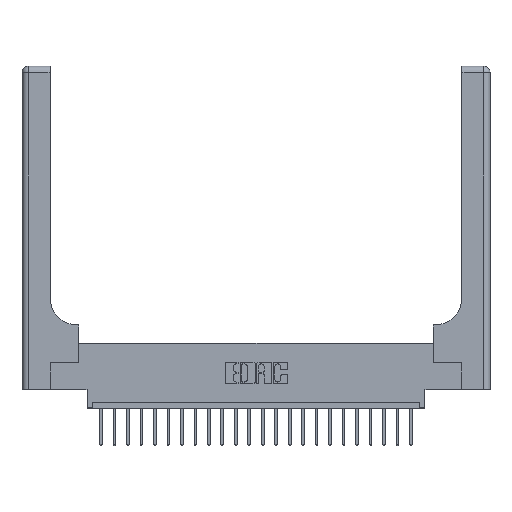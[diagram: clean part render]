
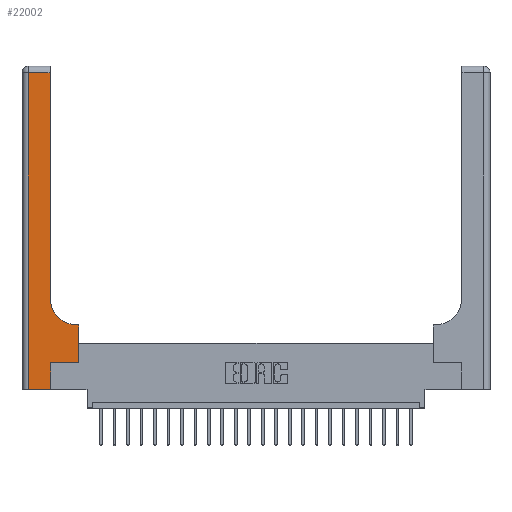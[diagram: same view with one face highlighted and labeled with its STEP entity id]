
A CAD part, top view. The second image highlights one B-rep face of the part: STEP entity #22002.
In plain terms, the highlighted planar face has unit normal (0, 0, 1).
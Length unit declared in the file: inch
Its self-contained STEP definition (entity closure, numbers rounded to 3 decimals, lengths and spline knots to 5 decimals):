
#860 = ORIENTED_EDGE ( 'NONE', *, *, #4540, .T. ) ;
#956 = ORIENTED_EDGE ( 'NONE', *, *, #17757, .T. ) ;
#1184 = EDGE_CURVE ( 'NONE', #16514, #21047, #18964, .T. ) ;
#1452 = CARTESIAN_POINT ( 'NONE',  ( 0.26, 3., 0.37 ) ) ;
#1758 = CARTESIAN_POINT ( 'NONE',  ( 0.528, 0.25, 0.37 ) ) ;
#2264 = DIRECTION ( 'NONE',  ( -1., 0., 0. ) ) ;
#2512 = CARTESIAN_POINT ( 'NONE',  ( 0.51, 0.85, 0.37 ) ) ;
#3030 = VERTEX_POINT ( 'NONE', #13563 ) ;
#3542 = DIRECTION ( 'NONE',  ( 0., 1., 0. ) ) ;
#3850 = EDGE_CURVE ( 'NONE', #17788, #13580, #21428, .T. ) ;
#3981 = CIRCLE ( 'NONE', #13680, 0.25 ) ;
#4122 = LINE ( 'NONE', #12991, #8092 ) ;
#4367 = DIRECTION ( 'NONE',  ( 1., 0., 0. ) ) ;
#4520 = ORIENTED_EDGE ( 'NONE', *, *, #20509, .T. ) ;
#4539 = EDGE_LOOP ( 'NONE', ( #12520, #20703, #9041, #860, #22827, #956, #18592, #10675, #4520 ) ) ;
#4540 = EDGE_CURVE ( 'NONE', #21047, #13183, #22746, .T. ) ;
#4977 = CARTESIAN_POINT ( 'NONE',  ( 0.528, 0.25, 0.37 ) ) ;
#5408 = DIRECTION ( 'NONE',  ( -1., 0., 0. ) ) ;
#5410 = CARTESIAN_POINT ( 'NONE',  ( 0.26, 0.6, 0.37 ) ) ;
#6060 = VECTOR ( 'NONE', #19617, 39.37008 ) ;
#6388 = DIRECTION ( 'NONE',  ( 1., 0., 0. ) ) ;
#7308 = VECTOR ( 'NONE', #6388, 39.37008 ) ;
#7372 = DIRECTION ( 'NONE',  ( 0., 1., 0. ) ) ;
#8092 = VECTOR ( 'NONE', #17781, 39.37008 ) ;
#8501 = AXIS2_PLACEMENT_3D ( 'NONE', #10665, #19775, #5408 ) ;
#8605 = CARTESIAN_POINT ( 'NONE',  ( 0., 0., 0.37 ) ) ;
#8743 = CARTESIAN_POINT ( 'NONE',  ( 0.528, 0.6, 0.37 ) ) ;
#9041 = ORIENTED_EDGE ( 'NONE', *, *, #1184, .T. ) ;
#10665 = CARTESIAN_POINT ( 'NONE',  ( 0., 3., 0.37 ) ) ;
#10675 = ORIENTED_EDGE ( 'NONE', *, *, #3850, .T. ) ;
#12109 = EDGE_CURVE ( 'NONE', #20172, #17788, #12489, .T. ) ;
#12306 = PLANE ( 'NONE',  #8501 ) ;
#12427 = VECTOR ( 'NONE', #7372, 39.37008 ) ;
#12489 = LINE ( 'NONE', #1758, #6060 ) ;
#12520 = ORIENTED_EDGE ( 'NONE', *, *, #20698, .T. ) ;
#12707 = CARTESIAN_POINT ( 'NONE',  ( 0.06, 2.94, 0.37 ) ) ;
#12991 = CARTESIAN_POINT ( 'NONE',  ( 0., 2.94, 0.37 ) ) ;
#13183 = VERTEX_POINT ( 'NONE', #19075 ) ;
#13563 = CARTESIAN_POINT ( 'NONE',  ( 0.26, 0.85, 0.37 ) ) ;
#13580 = VERTEX_POINT ( 'NONE', #21351 ) ;
#13680 = AXIS2_PLACEMENT_3D ( 'NONE', #2512, #20384, #4367 ) ;
#14725 = EDGE_CURVE ( 'NONE', #13183, #22139, #16025, .T. ) ;
#15343 = CARTESIAN_POINT ( 'NONE',  ( 0.06, 3., 0.37 ) ) ;
#15636 = LINE ( 'NONE', #22770, #21496 ) ;
#15750 = DIRECTION ( 'NONE',  ( 1., 0., 0. ) ) ;
#16025 = LINE ( 'NONE', #16253, #12427 ) ;
#16037 = FACE_OUTER_BOUND ( 'NONE', #4539, .T. ) ;
#16253 = CARTESIAN_POINT ( 'NONE',  ( 0.265, 0., 0.37 ) ) ;
#16514 = VERTEX_POINT ( 'NONE', #12707 ) ;
#16557 = CARTESIAN_POINT ( 'NONE',  ( 0.26, 2.94, 0.37 ) ) ;
#17088 = DIRECTION ( 'NONE',  ( 0., -1., 0. ) ) ;
#17695 = VECTOR ( 'NONE', #17088, 39.37008 ) ;
#17757 = EDGE_CURVE ( 'NONE', #22139, #20172, #15636, .T. ) ;
#17781 = DIRECTION ( 'NONE',  ( -1., 0., 0. ) ) ;
#17788 = VERTEX_POINT ( 'NONE', #8743 ) ;
#18592 = ORIENTED_EDGE ( 'NONE', *, *, #12109, .T. ) ;
#18782 = EDGE_CURVE ( 'NONE', #22976, #16514, #4122, .T. ) ;
#18902 = VECTOR ( 'NONE', #2264, 39.37008 ) ;
#18964 = LINE ( 'NONE', #15343, #17695 ) ;
#19075 = CARTESIAN_POINT ( 'NONE',  ( 0.265, 0., 0.37 ) ) ;
#19617 = DIRECTION ( 'NONE',  ( 0., 1., 0. ) ) ;
#19775 = DIRECTION ( 'NONE',  ( 0., 0., -1. ) ) ;
#20172 = VERTEX_POINT ( 'NONE', #4977 ) ;
#20384 = DIRECTION ( 'NONE',  ( 0., 0., -1. ) ) ;
#20509 = EDGE_CURVE ( 'NONE', #13580, #3030, #3981, .T. ) ;
#20698 = EDGE_CURVE ( 'NONE', #3030, #22976, #21070, .T. ) ;
#20703 = ORIENTED_EDGE ( 'NONE', *, *, #18782, .T. ) ;
#21047 = VERTEX_POINT ( 'NONE', #22105 ) ;
#21070 = LINE ( 'NONE', #1452, #22270 ) ;
#21351 = CARTESIAN_POINT ( 'NONE',  ( 0.51, 0.6, 0.37 ) ) ;
#21428 = LINE ( 'NONE', #5410, #18902 ) ;
#21496 = VECTOR ( 'NONE', #15750, 39.37008 ) ;
#22002 = ADVANCED_FACE ( 'NONE', ( #16037 ), #12306, .F. ) ;
#22105 = CARTESIAN_POINT ( 'NONE',  ( 0.06, 0., 0.37 ) ) ;
#22112 = CARTESIAN_POINT ( 'NONE',  ( 0.265, 0.25, 0.37 ) ) ;
#22139 = VERTEX_POINT ( 'NONE', #22112 ) ;
#22270 = VECTOR ( 'NONE', #3542, 39.37008 ) ;
#22746 = LINE ( 'NONE', #8605, #7308 ) ;
#22770 = CARTESIAN_POINT ( 'NONE',  ( 0.265, 0.25, 0.37 ) ) ;
#22827 = ORIENTED_EDGE ( 'NONE', *, *, #14725, .T. ) ;
#22976 = VERTEX_POINT ( 'NONE', #16557 ) ;
